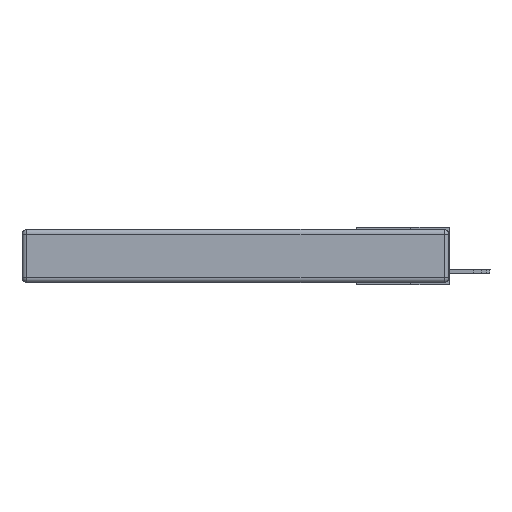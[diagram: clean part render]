
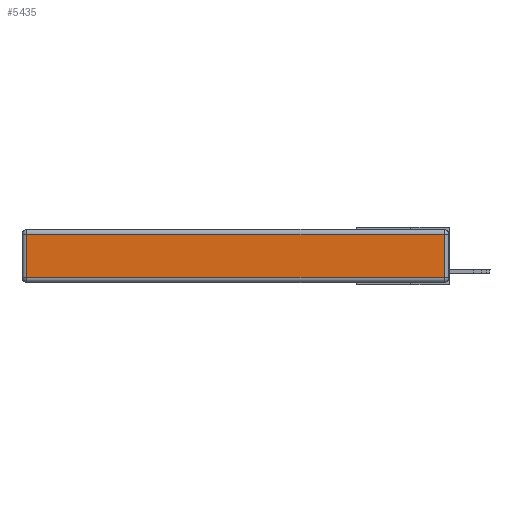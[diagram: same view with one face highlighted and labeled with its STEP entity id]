
A CAD part, left-side view. The second image highlights one B-rep face of the part: STEP entity #5435.
In plain terms, the highlighted planar face has unit normal (-1, 0, 0).
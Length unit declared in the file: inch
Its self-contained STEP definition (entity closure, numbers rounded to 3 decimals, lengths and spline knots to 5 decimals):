
#93 = LINE ( 'NONE', #4836, #1301 ) ;
#575 = VECTOR ( 'NONE', #15324, 39.37008 ) ;
#606 = VECTOR ( 'NONE', #20085, 39.37008 ) ;
#1301 = VECTOR ( 'NONE', #1512, 39.37008 ) ;
#1512 = DIRECTION ( 'NONE',  ( 0., 0., -1. ) ) ;
#1558 = VERTEX_POINT ( 'NONE', #2947 ) ;
#1563 = LINE ( 'NONE', #5756, #575 ) ;
#1871 = VERTEX_POINT ( 'NONE', #18745 ) ;
#2626 = LINE ( 'NONE', #16939, #606 ) ;
#2947 = CARTESIAN_POINT ( 'NONE',  ( 0., 0.03, -0.03 ) ) ;
#4836 = CARTESIAN_POINT ( 'NONE',  ( 0., 2.72, -0.343 ) ) ;
#4887 = CARTESIAN_POINT ( 'NONE',  ( 0., 2.72, -0.03 ) ) ;
#5435 = ADVANCED_FACE ( 'NONE', ( #20177 ), #16699, .T. ) ;
#5756 = CARTESIAN_POINT ( 'NONE',  ( 0., 0.03, -0.343 ) ) ;
#7079 = EDGE_CURVE ( 'NONE', #1558, #16649, #2626, .T. ) ;
#7762 = DIRECTION ( 'NONE',  ( 0., -1., 0. ) ) ;
#7928 = EDGE_LOOP ( 'NONE', ( #8217, #16670, #14913, #11222 ) ) ;
#8217 = ORIENTED_EDGE ( 'NONE', *, *, #13623, .T. ) ;
#8383 = CARTESIAN_POINT ( 'NONE',  ( 0., 0.03, -0.313 ) ) ;
#9243 = CARTESIAN_POINT ( 'NONE',  ( 0., 0., -0.313 ) ) ;
#11222 = ORIENTED_EDGE ( 'NONE', *, *, #17852, .T. ) ;
#11860 = DIRECTION ( 'NONE',  ( 0., 0., 1. ) ) ;
#11924 = CARTESIAN_POINT ( 'NONE',  ( 0., 0., -0.343 ) ) ;
#13315 = DIRECTION ( 'NONE',  ( -1., 0., 0. ) ) ;
#13455 = VECTOR ( 'NONE', #7762, 39.37008 ) ;
#13623 = EDGE_CURVE ( 'NONE', #1871, #19133, #17653, .T. ) ;
#14460 = EDGE_CURVE ( 'NONE', #19133, #1558, #1563, .T. ) ;
#14913 = ORIENTED_EDGE ( 'NONE', *, *, #7079, .T. ) ;
#15324 = DIRECTION ( 'NONE',  ( 0., 0., 1. ) ) ;
#16649 = VERTEX_POINT ( 'NONE', #4887 ) ;
#16670 = ORIENTED_EDGE ( 'NONE', *, *, #14460, .T. ) ;
#16699 = PLANE ( 'NONE',  #17620 ) ;
#16939 = CARTESIAN_POINT ( 'NONE',  ( 0., 2.75, -0.03 ) ) ;
#17620 = AXIS2_PLACEMENT_3D ( 'NONE', #11924, #13315, #11860 ) ;
#17653 = LINE ( 'NONE', #9243, #13455 ) ;
#17852 = EDGE_CURVE ( 'NONE', #16649, #1871, #93, .T. ) ;
#18745 = CARTESIAN_POINT ( 'NONE',  ( 0., 2.72, -0.313 ) ) ;
#19133 = VERTEX_POINT ( 'NONE', #8383 ) ;
#20085 = DIRECTION ( 'NONE',  ( 0., 1., 0. ) ) ;
#20177 = FACE_OUTER_BOUND ( 'NONE', #7928, .T. ) ;
